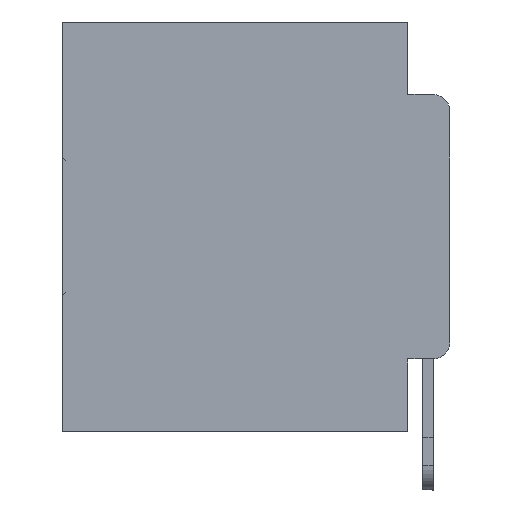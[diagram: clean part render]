
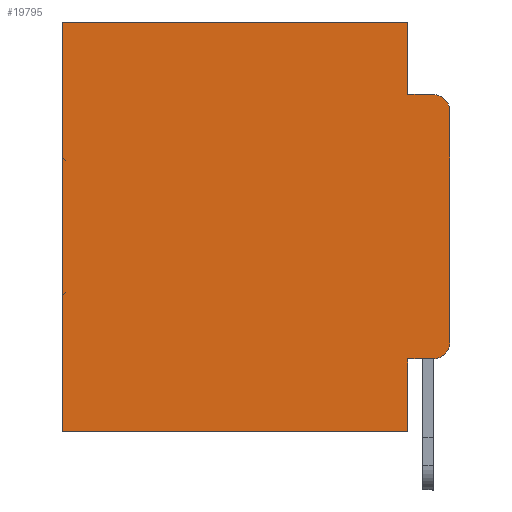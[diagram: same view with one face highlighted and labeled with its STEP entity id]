
A CAD part, left-side view. The second image highlights one B-rep face of the part: STEP entity #19795.
In plain terms, the highlighted planar face has unit normal (-1, 0, 0).
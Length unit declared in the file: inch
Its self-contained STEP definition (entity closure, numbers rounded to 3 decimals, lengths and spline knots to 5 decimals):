
#162 = CARTESIAN_POINT ( 'NONE',  ( 0.298, 0.051, 0. ) ) ;
#213 = CARTESIAN_POINT ( 'NONE',  ( 0.298, 0.02, -0.4115 ) ) ;
#412 = FACE_OUTER_BOUND ( 'NONE', #29215, .T. ) ;
#907 = ORIENTED_EDGE ( 'NONE', *, *, #21504, .F. ) ;
#1518 = EDGE_CURVE ( 'NONE', #9955, #16348, #6763, .T. ) ;
#2825 = VERTEX_POINT ( 'NONE', #4015 ) ;
#3248 = EDGE_CURVE ( 'NONE', #10396, #7736, #4303, .T. ) ;
#3664 = CARTESIAN_POINT ( 'NONE',  ( 0.298, 0.02, -0.1085 ) ) ;
#3971 = CARTESIAN_POINT ( 'NONE',  ( 0.298, 0.051, 0. ) ) ;
#4015 = CARTESIAN_POINT ( 'NONE',  ( 0.298, 0.473, 0. ) ) ;
#4303 = LINE ( 'NONE', #14258, #19666 ) ;
#5076 = CARTESIAN_POINT ( 'NONE',  ( 0.298, 0., 0. ) ) ;
#5156 = ORIENTED_EDGE ( 'NONE', *, *, #30452, .F. ) ;
#5404 = DIRECTION ( 'NONE',  ( 0., 0., -1. ) ) ;
#5746 = VERTEX_POINT ( 'NONE', #10887 ) ;
#6308 = CARTESIAN_POINT ( 'NONE',  ( 0.298, 0.051, -0.4115 ) ) ;
#6442 = VECTOR ( 'NONE', #5404, 39.37008 ) ;
#6763 = LINE ( 'NONE', #19228, #18654 ) ;
#7365 = DIRECTION ( 'NONE',  ( 0., 1., 0. ) ) ;
#7736 = VERTEX_POINT ( 'NONE', #9996 ) ;
#7780 = EDGE_CURVE ( 'NONE', #13954, #19659, #9513, .T. ) ;
#7834 = VECTOR ( 'NONE', #11772, 39.37008 ) ;
#8873 = LINE ( 'NONE', #3971, #25101 ) ;
#8876 = EDGE_CURVE ( 'NONE', #13954, #2825, #19673, .T. ) ;
#9297 = EDGE_CURVE ( 'NONE', #19659, #31505, #19487, .T. ) ;
#9513 = LINE ( 'NONE', #14576, #22918 ) ;
#9955 = VERTEX_POINT ( 'NONE', #6308 ) ;
#9996 = CARTESIAN_POINT ( 'NONE',  ( 0.298, 0., -0.3915 ) ) ;
#10396 = VERTEX_POINT ( 'NONE', #23002 ) ;
#10887 = CARTESIAN_POINT ( 'NONE',  ( 0.298, 0.473, -0.5 ) ) ;
#10999 = AXIS2_PLACEMENT_3D ( 'NONE', #28038, #25580, #30155 ) ;
#11772 = DIRECTION ( 'NONE',  ( 0., -1., 0. ) ) ;
#12543 = CIRCLE ( 'NONE', #13063, 0.02 ) ;
#12559 = EDGE_CURVE ( 'NONE', #2825, #5746, #21130, .T. ) ;
#12764 = LINE ( 'NONE', #22786, #23052 ) ;
#12838 = ORIENTED_EDGE ( 'NONE', *, *, #9297, .F. ) ;
#13063 = AXIS2_PLACEMENT_3D ( 'NONE', #3664, #13620, #23940 ) ;
#13620 = DIRECTION ( 'NONE',  ( -1., 0., 0. ) ) ;
#13954 = VERTEX_POINT ( 'NONE', #162 ) ;
#14258 = CARTESIAN_POINT ( 'NONE',  ( 0.298, 0., 0. ) ) ;
#14576 = CARTESIAN_POINT ( 'NONE',  ( 0.298, 0.051, 0. ) ) ;
#15246 = ORIENTED_EDGE ( 'NONE', *, *, #1518, .T. ) ;
#15555 = DIRECTION ( 'NONE',  ( -1., 0., 0. ) ) ;
#15694 = CARTESIAN_POINT ( 'NONE',  ( 0.298, 0.473, 0. ) ) ;
#16348 = VERTEX_POINT ( 'NONE', #213 ) ;
#17693 = DIRECTION ( 'NONE',  ( 0., 1., 0. ) ) ;
#17733 = PLANE ( 'NONE',  #10999 ) ;
#18601 = AXIS2_PLACEMENT_3D ( 'NONE', #25716, #15555, #28651 ) ;
#18654 = VECTOR ( 'NONE', #21858, 39.37008 ) ;
#19228 = CARTESIAN_POINT ( 'NONE',  ( 0.298, 0.051, -0.4115 ) ) ;
#19487 = LINE ( 'NONE', #24072, #7834 ) ;
#19659 = VERTEX_POINT ( 'NONE', #30319 ) ;
#19666 = VECTOR ( 'NONE', #24266, 39.37008 ) ;
#19673 = LINE ( 'NONE', #5076, #30282 ) ;
#19748 = CARTESIAN_POINT ( 'NONE',  ( 0.298, 0.02, -0.0885 ) ) ;
#19795 = ADVANCED_FACE ( 'NONE', ( #412 ), #17733, .F. ) ;
#19941 = EDGE_CURVE ( 'NONE', #10396, #31505, #12543, .T. ) ;
#20336 = CARTESIAN_POINT ( 'NONE',  ( 0.298, 0.051, -0.5 ) ) ;
#21130 = LINE ( 'NONE', #15694, #6442 ) ;
#21504 = EDGE_CURVE ( 'NONE', #27728, #5746, #12764, .T. ) ;
#21858 = DIRECTION ( 'NONE',  ( 0., -1., 0. ) ) ;
#22315 = DIRECTION ( 'NONE',  ( 0., 0., -1. ) ) ;
#22786 = CARTESIAN_POINT ( 'NONE',  ( 0.298, 0., -0.5 ) ) ;
#22918 = VECTOR ( 'NONE', #22315, 39.37008 ) ;
#23002 = CARTESIAN_POINT ( 'NONE',  ( 0.298, 0., -0.1085 ) ) ;
#23052 = VECTOR ( 'NONE', #17693, 39.37008 ) ;
#23701 = ORIENTED_EDGE ( 'NONE', *, *, #26588, .T. ) ;
#23940 = DIRECTION ( 'NONE',  ( 0., 0., -1. ) ) ;
#24072 = CARTESIAN_POINT ( 'NONE',  ( 0.298, 0.051, -0.0885 ) ) ;
#24187 = ORIENTED_EDGE ( 'NONE', *, *, #12559, .T. ) ;
#24266 = DIRECTION ( 'NONE',  ( 0., 0., -1. ) ) ;
#25101 = VECTOR ( 'NONE', #26380, 39.37008 ) ;
#25459 = ORIENTED_EDGE ( 'NONE', *, *, #19941, .T. ) ;
#25580 = DIRECTION ( 'NONE',  ( 1., 0., 0. ) ) ;
#25716 = CARTESIAN_POINT ( 'NONE',  ( 0.298, 0.02, -0.3915 ) ) ;
#25801 = ORIENTED_EDGE ( 'NONE', *, *, #7780, .F. ) ;
#26380 = DIRECTION ( 'NONE',  ( 0., 0., -1. ) ) ;
#26588 = EDGE_CURVE ( 'NONE', #16348, #7736, #27455, .T. ) ;
#26680 = ORIENTED_EDGE ( 'NONE', *, *, #3248, .F. ) ;
#27455 = CIRCLE ( 'NONE', #18601, 0.02 ) ;
#27530 = ORIENTED_EDGE ( 'NONE', *, *, #8876, .T. ) ;
#27728 = VERTEX_POINT ( 'NONE', #20336 ) ;
#28038 = CARTESIAN_POINT ( 'NONE',  ( 0.298, 0., 0. ) ) ;
#28651 = DIRECTION ( 'NONE',  ( 0., 0., -1. ) ) ;
#29215 = EDGE_LOOP ( 'NONE', ( #26680, #25459, #12838, #25801, #27530, #24187, #907, #5156, #15246, #23701 ) ) ;
#30155 = DIRECTION ( 'NONE',  ( 0., 0., -1. ) ) ;
#30282 = VECTOR ( 'NONE', #7365, 39.37008 ) ;
#30319 = CARTESIAN_POINT ( 'NONE',  ( 0.298, 0.051, -0.0885 ) ) ;
#30452 = EDGE_CURVE ( 'NONE', #9955, #27728, #8873, .T. ) ;
#31505 = VERTEX_POINT ( 'NONE', #19748 ) ;
